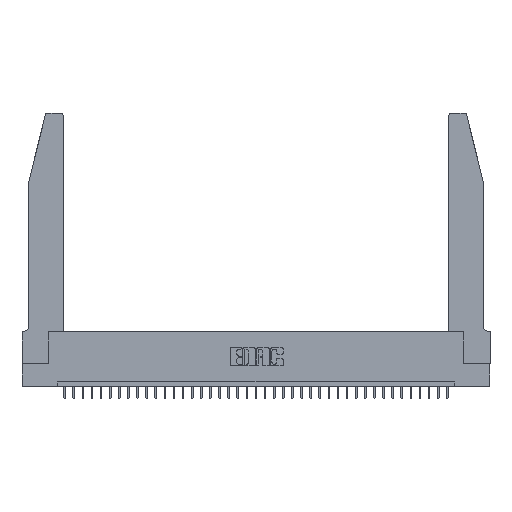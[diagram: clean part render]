
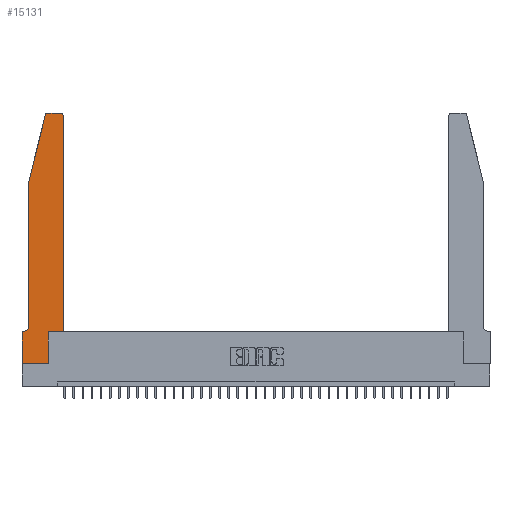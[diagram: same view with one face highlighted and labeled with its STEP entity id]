
A CAD part, top view. The second image highlights one B-rep face of the part: STEP entity #15131.
In plain terms, the highlighted planar face has unit normal (0, 0, 1).
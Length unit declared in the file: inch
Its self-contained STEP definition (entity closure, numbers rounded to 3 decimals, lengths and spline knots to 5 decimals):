
#106 = AXIS2_PLACEMENT_3D ( 'NONE', #6498, #475, #14947 ) ;
#344 = EDGE_CURVE ( 'NONE', #10673, #29617, #8751, .T. ) ;
#475 = DIRECTION ( 'NONE',  ( 0., 0., 1. ) ) ;
#561 = CARTESIAN_POINT ( 'NONE',  ( 0.4205, 2.72, 0.37 ) ) ;
#905 = EDGE_LOOP ( 'NONE', ( #25783, #11421, #30708, #25080, #2863, #16072, #18175, #4994, #15326, #4940, #1985, #19426 ) ) ;
#1627 = LINE ( 'NONE', #36135, #31171 ) ;
#1885 = VERTEX_POINT ( 'NONE', #6718 ) ;
#1985 = ORIENTED_EDGE ( 'NONE', *, *, #344, .T. ) ;
#2863 = ORIENTED_EDGE ( 'NONE', *, *, #8043, .T. ) ;
#3019 = VERTEX_POINT ( 'NONE', #11610 ) ;
#3294 = EDGE_CURVE ( 'NONE', #21536, #3019, #1627, .T. ) ;
#4843 = EDGE_CURVE ( 'NONE', #31206, #10673, #25167, .T. ) ;
#4940 = ORIENTED_EDGE ( 'NONE', *, *, #4843, .T. ) ;
#4994 = ORIENTED_EDGE ( 'NONE', *, *, #27925, .T. ) ;
#6241 = AXIS2_PLACEMENT_3D ( 'NONE', #561, #29262, #9411 ) ;
#6498 = CARTESIAN_POINT ( 'NONE',  ( 0., 0.35, 0.37 ) ) ;
#6718 = CARTESIAN_POINT ( 'NONE',  ( 0., 0., 0.37 ) ) ;
#6786 = DIRECTION ( 'NONE',  ( 0., 0., -1. ) ) ;
#6866 = CIRCLE ( 'NONE', #29612, 0.03 ) ;
#7234 = CARTESIAN_POINT ( 'NONE',  ( 0., 0., 0.37 ) ) ;
#7431 = CARTESIAN_POINT ( 'NONE',  ( 0.0755, 0.35, 0.37 ) ) ;
#8043 = EDGE_CURVE ( 'NONE', #3019, #20080, #12257, .T. ) ;
#8245 = EDGE_CURVE ( 'NONE', #35733, #26422, #6866, .T. ) ;
#8571 = FACE_OUTER_BOUND ( 'NONE', #905, .T. ) ;
#8751 = LINE ( 'NONE', #20189, #15532 ) ;
#9029 = CARTESIAN_POINT ( 'NONE',  ( 0.4205, 2.75, 0.37 ) ) ;
#9035 = CARTESIAN_POINT ( 'NONE',  ( 0.2865, 0.35, 0.37 ) ) ;
#9411 = DIRECTION ( 'NONE',  ( 1., 0., 0. ) ) ;
#9423 = DIRECTION ( 'NONE',  ( 1., 0., 0. ) ) ;
#9777 = VECTOR ( 'NONE', #18494, 39.37008 ) ;
#9864 = LINE ( 'NONE', #7234, #22724 ) ;
#9976 = CARTESIAN_POINT ( 'NONE',  ( 0.0055, 0.42, 0.37 ) ) ;
#10154 = DIRECTION ( 'NONE',  ( -1., 0., 0. ) ) ;
#10673 = VERTEX_POINT ( 'NONE', #23853 ) ;
#10739 = VECTOR ( 'NONE', #9423, 39.37008 ) ;
#11305 = DIRECTION ( 'NONE',  ( 0., 1., 0. ) ) ;
#11421 = ORIENTED_EDGE ( 'NONE', *, *, #8245, .T. ) ;
#11610 = CARTESIAN_POINT ( 'NONE',  ( 0.0755, 0.42, 0.37 ) ) ;
#12257 = CIRCLE ( 'NONE', #15851, 0.07 ) ;
#12731 = DIRECTION ( 'NONE',  ( -0.239, -0.971, 0. ) ) ;
#12929 = CARTESIAN_POINT ( 'NONE',  ( 0.4505, 2.72, 0.37 ) ) ;
#13498 = DIRECTION ( 'NONE',  ( 0., 1., 0. ) ) ;
#14691 = CARTESIAN_POINT ( 'NONE',  ( 0.2865, 0.35, 0.37 ) ) ;
#14947 = DIRECTION ( 'NONE',  ( 1., 0., 0. ) ) ;
#15131 = ADVANCED_FACE ( 'NONE', ( #8571 ), #22992, .T. ) ;
#15326 = ORIENTED_EDGE ( 'NONE', *, *, #19951, .T. ) ;
#15532 = VECTOR ( 'NONE', #13498, 39.37008 ) ;
#15851 = AXIS2_PLACEMENT_3D ( 'NONE', #9976, #6786, #10154 ) ;
#16072 = ORIENTED_EDGE ( 'NONE', *, *, #34582, .T. ) ;
#18175 = ORIENTED_EDGE ( 'NONE', *, *, #28971, .T. ) ;
#18374 = EDGE_CURVE ( 'NONE', #29617, #18416, #21201, .T. ) ;
#18416 = VERTEX_POINT ( 'NONE', #9029 ) ;
#18494 = DIRECTION ( 'NONE',  ( -1., 0., 0. ) ) ;
#19426 = ORIENTED_EDGE ( 'NONE', *, *, #18374, .T. ) ;
#19793 = CARTESIAN_POINT ( 'NONE',  ( 0.2605, 2.75, 0.37 ) ) ;
#19951 = EDGE_CURVE ( 'NONE', #35766, #31206, #36978, .T. ) ;
#20080 = VERTEX_POINT ( 'NONE', #30032 ) ;
#20189 = CARTESIAN_POINT ( 'NONE',  ( 0.4505, 0.35, 0.37 ) ) ;
#20707 = VECTOR ( 'NONE', #11305, 39.37008 ) ;
#21171 = LINE ( 'NONE', #26963, #34031 ) ;
#21201 = CIRCLE ( 'NONE', #6241, 0.03 ) ;
#21536 = VERTEX_POINT ( 'NONE', #26804 ) ;
#22724 = VECTOR ( 'NONE', #23923, 39.37008 ) ;
#22992 = PLANE ( 'NONE',  #106 ) ;
#23853 = CARTESIAN_POINT ( 'NONE',  ( 0.4505, 0.35, 0.37 ) ) ;
#23923 = DIRECTION ( 'NONE',  ( 0., -1., 0. ) ) ;
#24211 = EDGE_CURVE ( 'NONE', #26422, #21536, #21171, .T. ) ;
#24655 = VECTOR ( 'NONE', #36979, 39.37008 ) ;
#25080 = ORIENTED_EDGE ( 'NONE', *, *, #3294, .T. ) ;
#25167 = LINE ( 'NONE', #25532, #24655 ) ;
#25532 = CARTESIAN_POINT ( 'NONE',  ( 0.4505, 0.35, 0.37 ) ) ;
#25783 = ORIENTED_EDGE ( 'NONE', *, *, #34726, .T. ) ;
#26422 = VERTEX_POINT ( 'NONE', #28174 ) ;
#26804 = CARTESIAN_POINT ( 'NONE',  ( 0.0755, 2., 0.37 ) ) ;
#26961 = DIRECTION ( 'NONE',  ( 0., -1., 0. ) ) ;
#26963 = CARTESIAN_POINT ( 'NONE',  ( 0.0755, 2., 0.37 ) ) ;
#27567 = DIRECTION ( 'NONE',  ( 1., 0., 0. ) ) ;
#27925 = EDGE_CURVE ( 'NONE', #1885, #35766, #29098, .T. ) ;
#28174 = CARTESIAN_POINT ( 'NONE',  ( 0.25487, 2.72718, 0.37 ) ) ;
#28534 = CARTESIAN_POINT ( 'NONE',  ( 0.2865, 0., 0.37 ) ) ;
#28971 = EDGE_CURVE ( 'NONE', #37006, #1885, #9864, .T. ) ;
#29098 = LINE ( 'NONE', #34723, #10739 ) ;
#29262 = DIRECTION ( 'NONE',  ( 0., 0., 1. ) ) ;
#29612 = AXIS2_PLACEMENT_3D ( 'NONE', #36382, #33566, #27567 ) ;
#29617 = VERTEX_POINT ( 'NONE', #12929 ) ;
#29824 = CARTESIAN_POINT ( 'NONE',  ( 0., 0.35, 0.37 ) ) ;
#30032 = CARTESIAN_POINT ( 'NONE',  ( 0.0055, 0.35, 0.37 ) ) ;
#30121 = LINE ( 'NONE', #7431, #9777 ) ;
#30708 = ORIENTED_EDGE ( 'NONE', *, *, #24211, .T. ) ;
#31171 = VECTOR ( 'NONE', #26961, 39.37008 ) ;
#31206 = VERTEX_POINT ( 'NONE', #9035 ) ;
#31224 = DIRECTION ( 'NONE',  ( -1., 0., 0. ) ) ;
#33566 = DIRECTION ( 'NONE',  ( 0., 0., 1. ) ) ;
#33758 = VECTOR ( 'NONE', #31224, 39.37008 ) ;
#34031 = VECTOR ( 'NONE', #12731, 39.37008 ) ;
#34153 = CARTESIAN_POINT ( 'NONE',  ( 0.284, 2.75, 0.37 ) ) ;
#34221 = LINE ( 'NONE', #19793, #33758 ) ;
#34582 = EDGE_CURVE ( 'NONE', #20080, #37006, #30121, .T. ) ;
#34723 = CARTESIAN_POINT ( 'NONE',  ( 0., 0., 0.37 ) ) ;
#34726 = EDGE_CURVE ( 'NONE', #18416, #35733, #34221, .T. ) ;
#35733 = VERTEX_POINT ( 'NONE', #34153 ) ;
#35766 = VERTEX_POINT ( 'NONE', #28534 ) ;
#36135 = CARTESIAN_POINT ( 'NONE',  ( 0.0755, 2., 0.37 ) ) ;
#36382 = CARTESIAN_POINT ( 'NONE',  ( 0.284, 2.72, 0.37 ) ) ;
#36978 = LINE ( 'NONE', #14691, #20707 ) ;
#36979 = DIRECTION ( 'NONE',  ( 1., 0., 0. ) ) ;
#37006 = VERTEX_POINT ( 'NONE', #29824 ) ;
